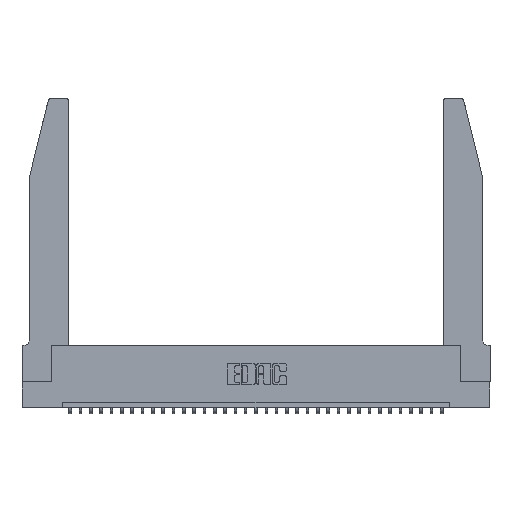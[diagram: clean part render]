
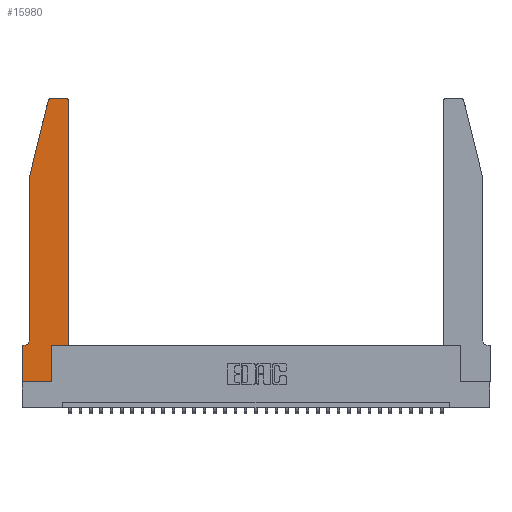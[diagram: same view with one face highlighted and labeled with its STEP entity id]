
A CAD part, top view. The second image highlights one B-rep face of the part: STEP entity #15980.
In plain terms, the highlighted planar face has unit normal (0, 0, 1).
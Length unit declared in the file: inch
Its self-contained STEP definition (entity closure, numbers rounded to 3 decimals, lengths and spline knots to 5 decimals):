
#40 = EDGE_CURVE ( 'NONE', #21568, #13302, #19307, .T. ) ;
#249 = EDGE_CURVE ( 'NONE', #19248, #25824, #29392, .T. ) ;
#742 = LINE ( 'NONE', #19738, #18866 ) ;
#839 = DIRECTION ( 'NONE',  ( 0., -1., 0. ) ) ;
#1103 = DIRECTION ( 'NONE',  ( -0.239, -0.971, 0. ) ) ;
#1140 = AXIS2_PLACEMENT_3D ( 'NONE', #16882, #21842, #1165 ) ;
#1165 = DIRECTION ( 'NONE',  ( 1., 0., 0. ) ) ;
#1599 = ORIENTED_EDGE ( 'NONE', *, *, #18574, .T. ) ;
#1642 = EDGE_CURVE ( 'NONE', #13302, #19248, #21208, .T. ) ;
#1820 = DIRECTION ( 'NONE',  ( 1., 0., 0. ) ) ;
#2157 = CARTESIAN_POINT ( 'NONE',  ( 0.2865, 0.35, 0.37 ) ) ;
#2210 = AXIS2_PLACEMENT_3D ( 'NONE', #31645, #29164, #13629 ) ;
#2306 = DIRECTION ( 'NONE',  ( 0., 1., 0. ) ) ;
#2325 = DIRECTION ( 'NONE',  ( 0., 1., 0. ) ) ;
#2343 = ORIENTED_EDGE ( 'NONE', *, *, #19173, .T. ) ;
#2822 = CARTESIAN_POINT ( 'NONE',  ( 0.4205, 2.75, 0.37 ) ) ;
#3246 = VERTEX_POINT ( 'NONE', #29423 ) ;
#3445 = VERTEX_POINT ( 'NONE', #6715 ) ;
#4290 = VECTOR ( 'NONE', #2325, 39.37008 ) ;
#4432 = ORIENTED_EDGE ( 'NONE', *, *, #30376, .T. ) ;
#4746 = CARTESIAN_POINT ( 'NONE',  ( 0., 0.35, 0.37 ) ) ;
#5009 = VERTEX_POINT ( 'NONE', #6390 ) ;
#5046 = ORIENTED_EDGE ( 'NONE', *, *, #249, .T. ) ;
#5710 = CARTESIAN_POINT ( 'NONE',  ( 0.0055, 0.35, 0.37 ) ) ;
#5812 = CARTESIAN_POINT ( 'NONE',  ( 0.25487, 2.72718, 0.37 ) ) ;
#6302 = EDGE_CURVE ( 'NONE', #25730, #20567, #32969, .T. ) ;
#6390 = CARTESIAN_POINT ( 'NONE',  ( 0.284, 2.75, 0.37 ) ) ;
#6470 = VECTOR ( 'NONE', #1820, 39.37008 ) ;
#6715 = CARTESIAN_POINT ( 'NONE',  ( 0.2865, 0., 0.37 ) ) ;
#6775 = VECTOR ( 'NONE', #24288, 39.37008 ) ;
#6888 = DIRECTION ( 'NONE',  ( 1., 0., 0. ) ) ;
#7278 = CARTESIAN_POINT ( 'NONE',  ( 0., 0., 0.37 ) ) ;
#7443 = CARTESIAN_POINT ( 'NONE',  ( 0.0055, 0.42, 0.37 ) ) ;
#7836 = ORIENTED_EDGE ( 'NONE', *, *, #40, .T. ) ;
#8190 = CARTESIAN_POINT ( 'NONE',  ( 0., 0., 0.37 ) ) ;
#8994 = CARTESIAN_POINT ( 'NONE',  ( 0.0755, 2., 0.37 ) ) ;
#9169 = VECTOR ( 'NONE', #2306, 39.37008 ) ;
#9744 = VECTOR ( 'NONE', #33155, 39.37008 ) ;
#9848 = CARTESIAN_POINT ( 'NONE',  ( 0.0755, 0.35, 0.37 ) ) ;
#11069 = CIRCLE ( 'NONE', #2210, 0.03 ) ;
#11310 = VECTOR ( 'NONE', #1103, 39.37008 ) ;
#11373 = EDGE_CURVE ( 'NONE', #24506, #25730, #24486, .T. ) ;
#11782 = EDGE_CURVE ( 'NONE', #24145, #3246, #17600, .T. ) ;
#13043 = DIRECTION ( 'NONE',  ( -1., 0., 0. ) ) ;
#13302 = VERTEX_POINT ( 'NONE', #25580 ) ;
#13629 = DIRECTION ( 'NONE',  ( 1., 0., 0. ) ) ;
#14190 = AXIS2_PLACEMENT_3D ( 'NONE', #32281, #19457, #6888 ) ;
#14802 = VECTOR ( 'NONE', #839, 39.37008 ) ;
#14944 = EDGE_CURVE ( 'NONE', #25824, #5009, #25005, .T. ) ;
#15939 = AXIS2_PLACEMENT_3D ( 'NONE', #7443, #23272, #13043 ) ;
#15980 = ADVANCED_FACE ( 'NONE', ( #33372 ), #19114, .T. ) ;
#16211 = ORIENTED_EDGE ( 'NONE', *, *, #20955, .T. ) ;
#16540 = ORIENTED_EDGE ( 'NONE', *, *, #6302, .T. ) ;
#16882 = CARTESIAN_POINT ( 'NONE',  ( 0.4205, 2.72, 0.37 ) ) ;
#16899 = DIRECTION ( 'NONE',  ( 1., 0., 0. ) ) ;
#17242 = ORIENTED_EDGE ( 'NONE', *, *, #11373, .T. ) ;
#17442 = DIRECTION ( 'NONE',  ( -1., 0., 0. ) ) ;
#17600 = LINE ( 'NONE', #21598, #6775 ) ;
#17758 = VERTEX_POINT ( 'NONE', #5812 ) ;
#17922 = CARTESIAN_POINT ( 'NONE',  ( 0.4505, 2.72, 0.37 ) ) ;
#18104 = EDGE_LOOP ( 'NONE', ( #29886, #16211, #4432, #26337, #1599, #17242, #16540, #19605, #2343, #7836, #32363, #5046 ) ) ;
#18574 = EDGE_CURVE ( 'NONE', #3246, #24506, #25975, .T. ) ;
#18866 = VECTOR ( 'NONE', #16899, 39.37008 ) ;
#19114 = PLANE ( 'NONE',  #14190 ) ;
#19173 = EDGE_CURVE ( 'NONE', #3445, #21568, #28053, .T. ) ;
#19248 = VERTEX_POINT ( 'NONE', #17922 ) ;
#19307 = LINE ( 'NONE', #30281, #6470 ) ;
#19437 = CARTESIAN_POINT ( 'NONE',  ( 0.0755, 2., 0.37 ) ) ;
#19457 = DIRECTION ( 'NONE',  ( 0., 0., 1. ) ) ;
#19605 = ORIENTED_EDGE ( 'NONE', *, *, #31268, .T. ) ;
#19738 = CARTESIAN_POINT ( 'NONE',  ( 0., 0., 0.37 ) ) ;
#20567 = VERTEX_POINT ( 'NONE', #7278 ) ;
#20641 = CARTESIAN_POINT ( 'NONE',  ( 0.2605, 2.75, 0.37 ) ) ;
#20955 = EDGE_CURVE ( 'NONE', #5009, #17758, #11069, .T. ) ;
#21208 = LINE ( 'NONE', #22763, #9169 ) ;
#21568 = VERTEX_POINT ( 'NONE', #2157 ) ;
#21598 = CARTESIAN_POINT ( 'NONE',  ( 0.0755, 2., 0.37 ) ) ;
#21842 = DIRECTION ( 'NONE',  ( 0., 0., 1. ) ) ;
#22763 = CARTESIAN_POINT ( 'NONE',  ( 0.4505, 0.35, 0.37 ) ) ;
#23272 = DIRECTION ( 'NONE',  ( 0., 0., -1. ) ) ;
#24145 = VERTEX_POINT ( 'NONE', #19437 ) ;
#24288 = DIRECTION ( 'NONE',  ( 0., -1., 0. ) ) ;
#24486 = LINE ( 'NONE', #9848, #30938 ) ;
#24506 = VERTEX_POINT ( 'NONE', #5710 ) ;
#25005 = LINE ( 'NONE', #20641, #9744 ) ;
#25580 = CARTESIAN_POINT ( 'NONE',  ( 0.4505, 0.35, 0.37 ) ) ;
#25730 = VERTEX_POINT ( 'NONE', #4746 ) ;
#25776 = LINE ( 'NONE', #8994, #11310 ) ;
#25824 = VERTEX_POINT ( 'NONE', #2822 ) ;
#25975 = CIRCLE ( 'NONE', #15939, 0.07 ) ;
#26337 = ORIENTED_EDGE ( 'NONE', *, *, #11782, .T. ) ;
#27741 = CARTESIAN_POINT ( 'NONE',  ( 0.2865, 0.35, 0.37 ) ) ;
#28053 = LINE ( 'NONE', #27741, #4290 ) ;
#29164 = DIRECTION ( 'NONE',  ( 0., 0., 1. ) ) ;
#29392 = CIRCLE ( 'NONE', #1140, 0.03 ) ;
#29423 = CARTESIAN_POINT ( 'NONE',  ( 0.0755, 0.42, 0.37 ) ) ;
#29886 = ORIENTED_EDGE ( 'NONE', *, *, #14944, .T. ) ;
#30281 = CARTESIAN_POINT ( 'NONE',  ( 0.4505, 0.35, 0.37 ) ) ;
#30376 = EDGE_CURVE ( 'NONE', #17758, #24145, #25776, .T. ) ;
#30938 = VECTOR ( 'NONE', #17442, 39.37008 ) ;
#31268 = EDGE_CURVE ( 'NONE', #20567, #3445, #742, .T. ) ;
#31645 = CARTESIAN_POINT ( 'NONE',  ( 0.284, 2.72, 0.37 ) ) ;
#32281 = CARTESIAN_POINT ( 'NONE',  ( 0., 0.35, 0.37 ) ) ;
#32363 = ORIENTED_EDGE ( 'NONE', *, *, #1642, .T. ) ;
#32969 = LINE ( 'NONE', #8190, #14802 ) ;
#33155 = DIRECTION ( 'NONE',  ( -1., 0., 0. ) ) ;
#33372 = FACE_OUTER_BOUND ( 'NONE', #18104, .T. ) ;
